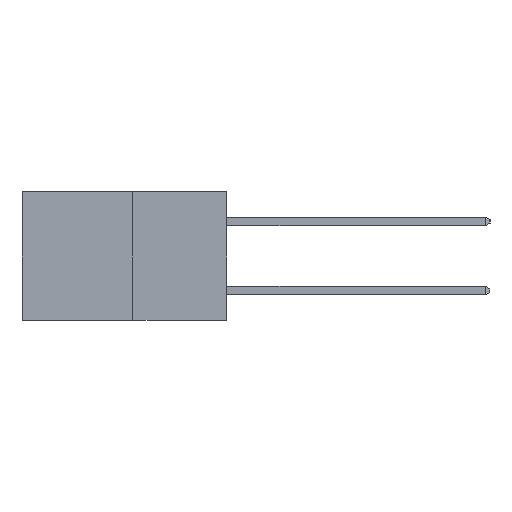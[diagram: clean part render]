
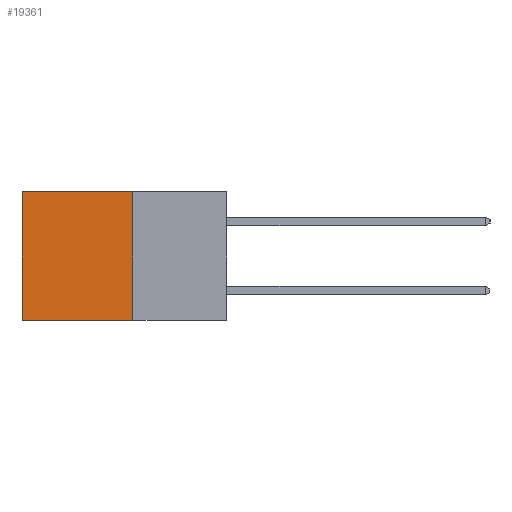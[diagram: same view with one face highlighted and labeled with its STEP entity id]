
A CAD part, left-side view. The second image highlights one B-rep face of the part: STEP entity #19361.
In plain terms, the highlighted planar face has unit normal (-1, 0, 0).
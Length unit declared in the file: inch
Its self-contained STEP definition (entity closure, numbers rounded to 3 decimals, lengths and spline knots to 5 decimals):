
#1054 = VECTOR ( 'NONE', #11654, 39.37008 ) ;
#1104 = DIRECTION ( 'NONE',  ( 0., 0., -1. ) ) ;
#1258 = FACE_OUTER_BOUND ( 'NONE', #1771, .T. ) ;
#1771 = EDGE_LOOP ( 'NONE', ( #20144, #9049, #20020, #4213 ) ) ;
#2848 = VECTOR ( 'NONE', #6862, 39.37008 ) ;
#4213 = ORIENTED_EDGE ( 'NONE', *, *, #14796, .T. ) ;
#4513 = VECTOR ( 'NONE', #1104, 39.37008 ) ;
#5167 = CARTESIAN_POINT ( 'NONE',  ( 0.277, 0.27, 0. ) ) ;
#5443 = EDGE_CURVE ( 'NONE', #16611, #8407, #10127, .T. ) ;
#5558 = DIRECTION ( 'NONE',  ( 1., 0., 0. ) ) ;
#6862 = DIRECTION ( 'NONE',  ( 0., 1., 0. ) ) ;
#7055 = EDGE_CURVE ( 'NONE', #8407, #13918, #20820, .T. ) ;
#7441 = CARTESIAN_POINT ( 'NONE',  ( 0.277, 0.59, -0.37 ) ) ;
#7663 = EDGE_CURVE ( 'NONE', #9976, #13918, #14381, .T. ) ;
#8407 = VERTEX_POINT ( 'NONE', #20088 ) ;
#9049 = ORIENTED_EDGE ( 'NONE', *, *, #7055, .F. ) ;
#9976 = VERTEX_POINT ( 'NONE', #18659 ) ;
#10127 = LINE ( 'NONE', #11469, #1054 ) ;
#11469 = CARTESIAN_POINT ( 'NONE',  ( 0.277, 0.27, -0.37 ) ) ;
#11511 = DIRECTION ( 'NONE',  ( 0., 1., 0. ) ) ;
#11654 = DIRECTION ( 'NONE',  ( 0., 0., -1. ) ) ;
#12206 = CARTESIAN_POINT ( 'NONE',  ( 0.277, 0.27, -0.37 ) ) ;
#13918 = VERTEX_POINT ( 'NONE', #19606 ) ;
#14381 = LINE ( 'NONE', #7441, #4513 ) ;
#14796 = EDGE_CURVE ( 'NONE', #16611, #9976, #16193, .T. ) ;
#15470 = PLANE ( 'NONE',  #17381 ) ;
#16193 = LINE ( 'NONE', #5167, #2848 ) ;
#16485 = VECTOR ( 'NONE', #11511, 39.37008 ) ;
#16611 = VERTEX_POINT ( 'NONE', #21504 ) ;
#17137 = DIRECTION ( 'NONE',  ( 0., 0., -1. ) ) ;
#17381 = AXIS2_PLACEMENT_3D ( 'NONE', #12206, #5558, #17137 ) ;
#18659 = CARTESIAN_POINT ( 'NONE',  ( 0.277, 0.59, 0. ) ) ;
#18778 = CARTESIAN_POINT ( 'NONE',  ( 0.277, 0.27, -0.37 ) ) ;
#19361 = ADVANCED_FACE ( 'NONE', ( #1258 ), #15470, .F. ) ;
#19606 = CARTESIAN_POINT ( 'NONE',  ( 0.277, 0.59, -0.37 ) ) ;
#20020 = ORIENTED_EDGE ( 'NONE', *, *, #5443, .F. ) ;
#20088 = CARTESIAN_POINT ( 'NONE',  ( 0.277, 0.27, -0.37 ) ) ;
#20144 = ORIENTED_EDGE ( 'NONE', *, *, #7663, .T. ) ;
#20820 = LINE ( 'NONE', #18778, #16485 ) ;
#21504 = CARTESIAN_POINT ( 'NONE',  ( 0.277, 0.27, 0. ) ) ;
